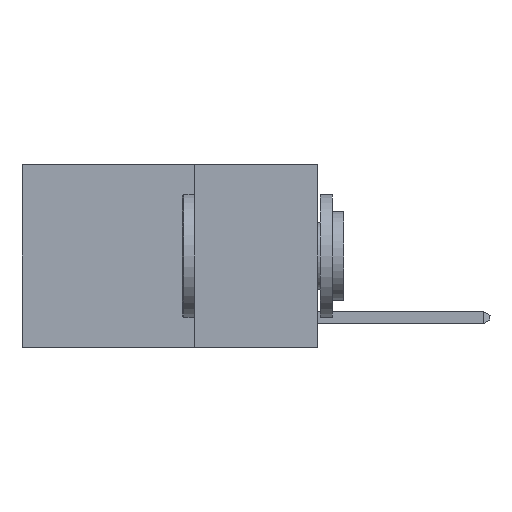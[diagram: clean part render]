
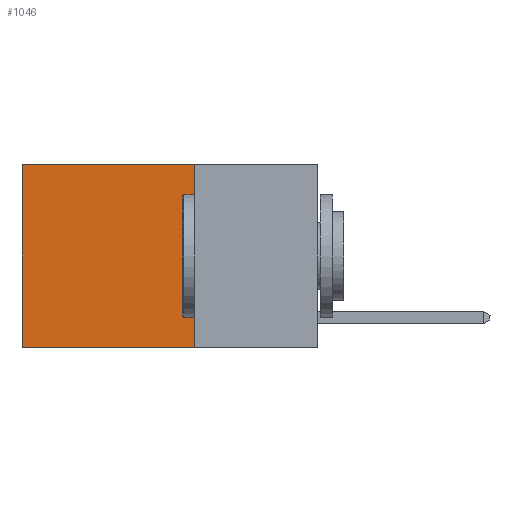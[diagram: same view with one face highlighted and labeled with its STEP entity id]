
A CAD part, left-side view. The second image highlights one B-rep face of the part: STEP entity #1046.
In plain terms, the highlighted planar face has unit normal (-1, 0, 0).
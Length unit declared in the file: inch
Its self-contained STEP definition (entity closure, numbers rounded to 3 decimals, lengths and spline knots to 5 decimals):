
#157 = CARTESIAN_POINT ( 'NONE',  ( 0.2625, 0.25, -0.37 ) ) ;
#443 = EDGE_CURVE ( 'NONE', #8826, #6236, #4719, .T. ) ;
#589 = CARTESIAN_POINT ( 'NONE',  ( 0.2625, 0.25, 0. ) ) ;
#662 = ORIENTED_EDGE ( 'NONE', *, *, #443, .T. ) ;
#825 = CARTESIAN_POINT ( 'NONE',  ( 0.2625, 0.25, 0. ) ) ;
#1046 = ADVANCED_FACE ( 'NONE', ( #10096 ), #1451, .F. ) ;
#1252 = VECTOR ( 'NONE', #5600, 39.37008 ) ;
#1451 = PLANE ( 'NONE',  #2516 ) ;
#1735 = LINE ( 'NONE', #157, #1252 ) ;
#2444 = CARTESIAN_POINT ( 'NONE',  ( 0.2625, 0.25, 0. ) ) ;
#2497 = EDGE_CURVE ( 'NONE', #7130, #8826, #8648, .T. ) ;
#2516 = AXIS2_PLACEMENT_3D ( 'NONE', #825, #10224, #4646 ) ;
#2610 = VECTOR ( 'NONE', #4056, 39.37008 ) ;
#3249 = CARTESIAN_POINT ( 'NONE',  ( 0.2625, 0.25, 0. ) ) ;
#3374 = ORIENTED_EDGE ( 'NONE', *, *, #7127, .F. ) ;
#3468 = VECTOR ( 'NONE', #4524, 39.37008 ) ;
#4056 = DIRECTION ( 'NONE',  ( 0., 0., -1. ) ) ;
#4103 = DIRECTION ( 'NONE',  ( 0., 0., -1. ) ) ;
#4524 = DIRECTION ( 'NONE',  ( 0., 1., 0. ) ) ;
#4646 = DIRECTION ( 'NONE',  ( 0., 0., -1. ) ) ;
#4719 = LINE ( 'NONE', #5457, #2610 ) ;
#5457 = CARTESIAN_POINT ( 'NONE',  ( 0.2625, 0.6, 0. ) ) ;
#5600 = DIRECTION ( 'NONE',  ( 0., 1., 0. ) ) ;
#5688 = CARTESIAN_POINT ( 'NONE',  ( 0.2625, 0.6, -0.37 ) ) ;
#6086 = ORIENTED_EDGE ( 'NONE', *, *, #6918, .F. ) ;
#6236 = VERTEX_POINT ( 'NONE', #5688 ) ;
#6918 = EDGE_CURVE ( 'NONE', #7108, #6236, #1735, .T. ) ;
#7108 = VERTEX_POINT ( 'NONE', #7878 ) ;
#7127 = EDGE_CURVE ( 'NONE', #7130, #7108, #9129, .T. ) ;
#7130 = VERTEX_POINT ( 'NONE', #3249 ) ;
#7674 = EDGE_LOOP ( 'NONE', ( #662, #6086, #3374, #8692 ) ) ;
#7878 = CARTESIAN_POINT ( 'NONE',  ( 0.2625, 0.25, -0.37 ) ) ;
#8648 = LINE ( 'NONE', #589, #3468 ) ;
#8692 = ORIENTED_EDGE ( 'NONE', *, *, #2497, .T. ) ;
#8826 = VERTEX_POINT ( 'NONE', #9717 ) ;
#8995 = VECTOR ( 'NONE', #4103, 39.37008 ) ;
#9129 = LINE ( 'NONE', #2444, #8995 ) ;
#9717 = CARTESIAN_POINT ( 'NONE',  ( 0.2625, 0.6, 0. ) ) ;
#10096 = FACE_OUTER_BOUND ( 'NONE', #7674, .T. ) ;
#10224 = DIRECTION ( 'NONE',  ( 1., 0., 0. ) ) ;
